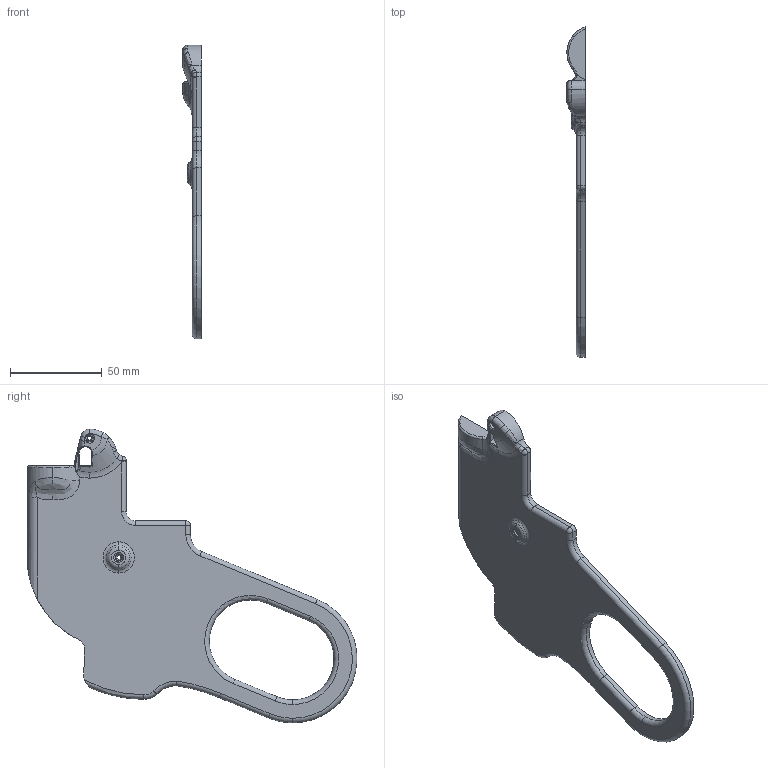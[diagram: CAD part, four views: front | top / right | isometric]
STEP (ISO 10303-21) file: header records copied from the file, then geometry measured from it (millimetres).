
FILE_DESCRIPTION (( 'STEP AP214' ), '1' );
FILE_NAME ('Side_Right.step', '2013-11-06T14:31:21', ( 'elpi' ), ( '' ), 'SwSTEP 2.0', 'SolidWorks 2013', '' );
FILE_SCHEMA (( 'AUTOMOTIVE_DESIGN' ));
Length unit declared in the file: millimetre
Products named in the file (1): Side_Right
Bounding box: 10 x 180.03 x 160.27 mm (x, y, z)
Volume: 62558 mm3; surface area: 29463 mm2
Topology: 1 solids, 1 shells, 192 faces, 603 edges, 374 vertices
Faces by surface type: cylinder 51, torus 38, sphere 37, bspline 36, plane 26, cone 4
Entity records: 7084 total; most frequent: CARTESIAN_POINT 2642, DIRECTION 935, ORIENTED_EDGE 916, EDGE_CURVE 458, AXIS2_PLACEMENT_3D 414, VERTEX_POINT 304, CIRCLE 257, EDGE_LOOP 236
